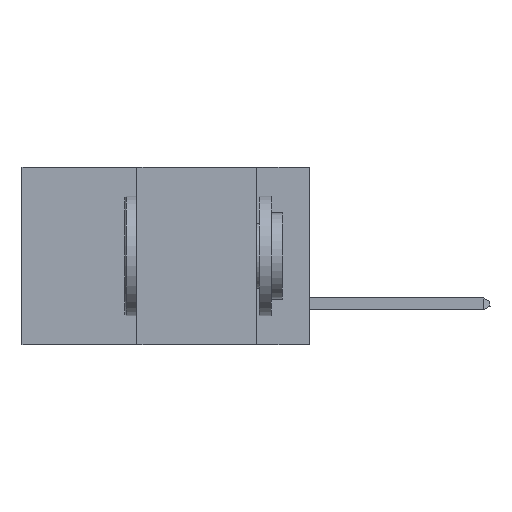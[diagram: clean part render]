
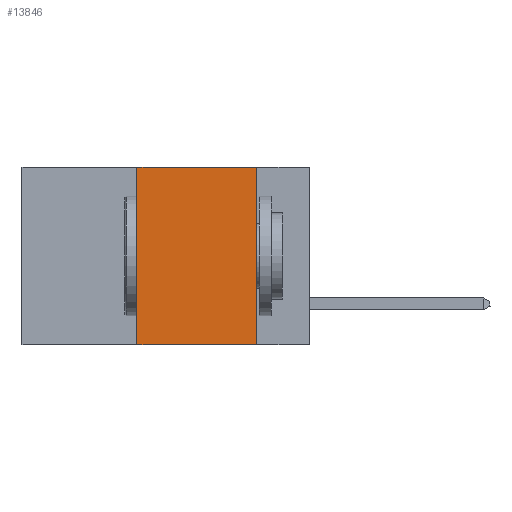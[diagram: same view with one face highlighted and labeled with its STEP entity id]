
A CAD part, left-side view. The second image highlights one B-rep face of the part: STEP entity #13846.
In plain terms, the highlighted planar face has unit normal (-1, 0, 0).
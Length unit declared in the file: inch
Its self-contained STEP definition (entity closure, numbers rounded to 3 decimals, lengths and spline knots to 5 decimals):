
#743 = ORIENTED_EDGE ( 'NONE', *, *, #12081, .F. ) ;
#1111 = CARTESIAN_POINT ( 'NONE',  ( 0., 0.6, 0. ) ) ;
#1479 = CARTESIAN_POINT ( 'NONE',  ( 0., 0.6, 0. ) ) ;
#2145 = DIRECTION ( 'NONE',  ( 0., 0., -1. ) ) ;
#2327 = VERTEX_POINT ( 'NONE', #12705 ) ;
#2653 = VECTOR ( 'NONE', #10902, 39.37008 ) ;
#2827 = EDGE_CURVE ( 'NONE', #4597, #9726, #7592, .T. ) ;
#3323 = ORIENTED_EDGE ( 'NONE', *, *, #11137, .T. ) ;
#4199 = DIRECTION ( 'NONE',  ( 0., -1., 0. ) ) ;
#4597 = VERTEX_POINT ( 'NONE', #11614 ) ;
#5867 = DIRECTION ( 'NONE',  ( 1., 0., 0. ) ) ;
#5939 = DIRECTION ( 'NONE',  ( 0., 0., -1. ) ) ;
#6902 = PLANE ( 'NONE',  #13657 ) ;
#7592 = LINE ( 'NONE', #13800, #2653 ) ;
#8069 = ORIENTED_EDGE ( 'NONE', *, *, #2827, .F. ) ;
#8306 = EDGE_LOOP ( 'NONE', ( #14474, #743, #8069, #3323 ) ) ;
#8546 = VECTOR ( 'NONE', #9474, 39.37008 ) ;
#8935 = LINE ( 'NONE', #9317, #14731 ) ;
#9317 = CARTESIAN_POINT ( 'NONE',  ( 0., 0.6, -0.37 ) ) ;
#9377 = VECTOR ( 'NONE', #5939, 39.37008 ) ;
#9405 = FACE_OUTER_BOUND ( 'NONE', #8306, .T. ) ;
#9474 = DIRECTION ( 'NONE',  ( 0., -1., 0. ) ) ;
#9726 = VERTEX_POINT ( 'NONE', #13860 ) ;
#10902 = DIRECTION ( 'NONE',  ( 0., 0., 1. ) ) ;
#11137 = EDGE_CURVE ( 'NONE', #4597, #2327, #8935, .T. ) ;
#11393 = CARTESIAN_POINT ( 'NONE',  ( 0., 0.11, 0. ) ) ;
#11614 = CARTESIAN_POINT ( 'NONE',  ( 0., 0.36, -0.37 ) ) ;
#11676 = LINE ( 'NONE', #1479, #8546 ) ;
#12081 = EDGE_CURVE ( 'NONE', #9726, #14865, #11676, .T. ) ;
#12460 = LINE ( 'NONE', #12832, #9377 ) ;
#12705 = CARTESIAN_POINT ( 'NONE',  ( 0., 0.11, -0.37 ) ) ;
#12832 = CARTESIAN_POINT ( 'NONE',  ( 0., 0.11, 0. ) ) ;
#13657 = AXIS2_PLACEMENT_3D ( 'NONE', #1111, #5867, #2145 ) ;
#13800 = CARTESIAN_POINT ( 'NONE',  ( 0., 0.36, 0. ) ) ;
#13846 = ADVANCED_FACE ( 'NONE', ( #9405 ), #6902, .F. ) ;
#13860 = CARTESIAN_POINT ( 'NONE',  ( 0., 0.36, 0. ) ) ;
#14474 = ORIENTED_EDGE ( 'NONE', *, *, #14980, .F. ) ;
#14731 = VECTOR ( 'NONE', #4199, 39.37008 ) ;
#14865 = VERTEX_POINT ( 'NONE', #11393 ) ;
#14980 = EDGE_CURVE ( 'NONE', #14865, #2327, #12460, .T. ) ;
